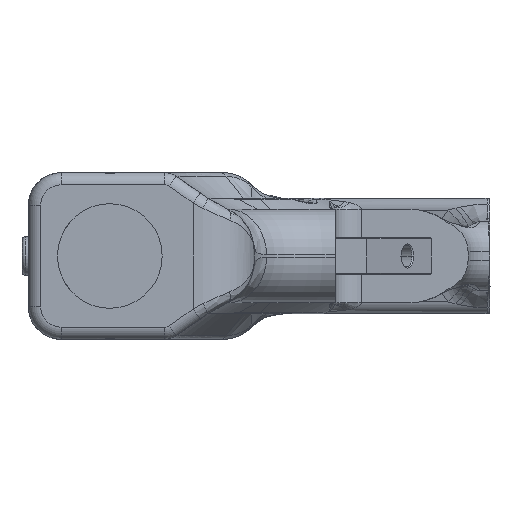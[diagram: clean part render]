
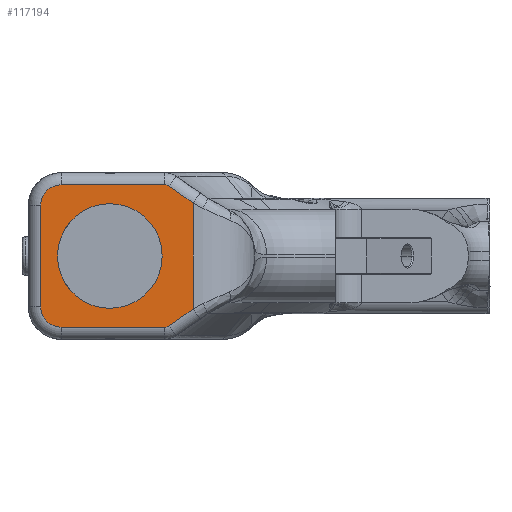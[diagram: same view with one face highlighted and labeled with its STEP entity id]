
A CAD part, left-side view. The second image highlights one B-rep face of the part: STEP entity #117194.
In plain terms, the highlighted planar face has unit normal (-1, 0, 0).
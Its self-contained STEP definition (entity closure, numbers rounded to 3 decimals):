
#360 = DIRECTION ( 'NONE',  ( 0., 0., 1. ) ) ;
#1329 = LINE ( 'NONE', #1911, #47660 ) ;
#1911 = CARTESIAN_POINT ( 'NONE',  ( -114.956, 0., -17.5 ) ) ;
#2619 = ORIENTED_EDGE ( 'NONE', *, *, #18241, .T. ) ;
#3771 = VECTOR ( 'NONE', #27679, 1000. ) ;
#4796 = ORIENTED_EDGE ( 'NONE', *, *, #19555, .T. ) ;
#6329 = CARTESIAN_POINT ( 'NONE',  ( -114.956, 105.1, -12.5 ) ) ;
#7355 = ORIENTED_EDGE ( 'NONE', *, *, #96632, .F. ) ;
#7951 = AXIS2_PLACEMENT_3D ( 'NONE', #50968, #42024, #105736 ) ;
#9005 = CARTESIAN_POINT ( 'NONE',  ( -114.956, 0., 20.5 ) ) ;
#9691 = ORIENTED_EDGE ( 'NONE', *, *, #30920, .T. ) ;
#10786 = CARTESIAN_POINT ( 'NONE',  ( -114.956, 69.321, -14.243 ) ) ;
#11739 = CARTESIAN_POINT ( 'NONE',  ( -114.956, 100.1, 12.5 ) ) ;
#11894 = CIRCLE ( 'NONE', #78513, 5. ) ;
#12187 = CIRCLE ( 'NONE', #109183, 12.875 ) ;
#14694 = LINE ( 'NONE', #106394, #98875 ) ;
#15686 = VECTOR ( 'NONE', #18559, 1000. ) ;
#16427 = ORIENTED_EDGE ( 'NONE', *, *, #97633, .F. ) ;
#16458 = DIRECTION ( 'NONE',  ( 0., 0., -1. ) ) ;
#16618 = AXIS2_PLACEMENT_3D ( 'NONE', #9005, #44818, #107895 ) ;
#17381 = ORIENTED_EDGE ( 'NONE', *, *, #26179, .T. ) ;
#17707 = DIRECTION ( 'NONE',  ( -1., 0., 0. ) ) ;
#18241 = EDGE_CURVE ( 'NONE', #76110, #98647, #51787, .T. ) ;
#18559 = DIRECTION ( 'NONE',  ( 0., -0.819, 0.574 ) ) ;
#19555 = EDGE_CURVE ( 'NONE', #110457, #112141, #101344, .T. ) ;
#22358 = DIRECTION ( 'NONE',  ( 0., 0., 1. ) ) ;
#22419 = DIRECTION ( 'NONE',  ( -1., 0., 0. ) ) ;
#26179 = EDGE_CURVE ( 'NONE', #66870, #110457, #110592, .T. ) ;
#26404 = CARTESIAN_POINT ( 'NONE',  ( -114.956, 74.602, -17.5 ) ) ;
#27619 = CARTESIAN_POINT ( 'NONE',  ( -114.956, 67.6, 13.038 ) ) ;
#27635 = ORIENTED_EDGE ( 'NONE', *, *, #94791, .F. ) ;
#27679 = DIRECTION ( 'NONE',  ( 0., 1., 0. ) ) ;
#28690 = CIRCLE ( 'NONE', #49685, 12.875 ) ;
#30236 = LINE ( 'NONE', #49335, #41963 ) ;
#30920 = EDGE_CURVE ( 'NONE', #75499, #31931, #11894, .T. ) ;
#31931 = VERTEX_POINT ( 'NONE', #103883 ) ;
#33222 = ORIENTED_EDGE ( 'NONE', *, *, #55880, .T. ) ;
#36606 = LINE ( 'NONE', #72950, #3771 ) ;
#37031 = CARTESIAN_POINT ( 'NONE',  ( -114.956, 88.1, 12.875 ) ) ;
#38508 = CARTESIAN_POINT ( 'NONE',  ( -114.956, 88.1, 0. ) ) ;
#38615 = DIRECTION ( 'NONE',  ( 0., 0.819, 0.574 ) ) ;
#40688 = LINE ( 'NONE', #41837, #67147 ) ;
#41305 = DIRECTION ( 'NONE',  ( -1., 0., 0. ) ) ;
#41555 = EDGE_CURVE ( 'NONE', #98647, #66870, #1329, .T. ) ;
#41837 = CARTESIAN_POINT ( 'NONE',  ( -114.956, 105.1, 20.5 ) ) ;
#41963 = VECTOR ( 'NONE', #38615, 1000. ) ;
#42024 = DIRECTION ( 'NONE',  ( -1., 0., 0. ) ) ;
#42637 = CARTESIAN_POINT ( 'NONE',  ( -114.956, 88.1, -12.875 ) ) ;
#44818 = DIRECTION ( 'NONE',  ( 1., 0., 0. ) ) ;
#46536 = EDGE_CURVE ( 'NONE', #31931, #76110, #40688, .T. ) ;
#47660 = VECTOR ( 'NONE', #100260, 1000. ) ;
#49335 = CARTESIAN_POINT ( 'NONE',  ( -114.956, 73.455, 17.138 ) ) ;
#49685 = AXIS2_PLACEMENT_3D ( 'NONE', #38508, #17707, #360 ) ;
#50829 = ORIENTED_EDGE ( 'NONE', *, *, #86669, .T. ) ;
#50968 = CARTESIAN_POINT ( 'NONE',  ( -114.956, 100.1, -12.5 ) ) ;
#51787 = CIRCLE ( 'NONE', #7951, 5. ) ;
#52511 = VERTEX_POINT ( 'NONE', #42637 ) ;
#54328 = FACE_OUTER_BOUND ( 'NONE', #108812, .T. ) ;
#55880 = EDGE_CURVE ( 'NONE', #89322, #75499, #36606, .T. ) ;
#56351 = VERTEX_POINT ( 'NONE', #95979 ) ;
#58770 = DIRECTION ( 'NONE',  ( 0., 0., -1. ) ) ;
#58804 = EDGE_LOOP ( 'NONE', ( #27635, #7355 ) ) ;
#65237 = ORIENTED_EDGE ( 'NONE', *, *, #41555, .T. ) ;
#66530 = DIRECTION ( 'NONE',  ( 0., 0., -1. ) ) ;
#66870 = VERTEX_POINT ( 'NONE', #26404 ) ;
#67147 = VECTOR ( 'NONE', #113297, 1000. ) ;
#67703 = CARTESIAN_POINT ( 'NONE',  ( -114.956, 74.602, 17.5 ) ) ;
#69094 = VERTEX_POINT ( 'NONE', #27619 ) ;
#71618 = FACE_BOUND ( 'NONE', #58804, .T. ) ;
#72950 = CARTESIAN_POINT ( 'NONE',  ( -114.956, 100.1, 17.5 ) ) ;
#73690 = CARTESIAN_POINT ( 'NONE',  ( -114.956, 100.1, 17.5 ) ) ;
#75499 = VERTEX_POINT ( 'NONE', #73690 ) ;
#76110 = VERTEX_POINT ( 'NONE', #6329 ) ;
#77280 = CIRCLE ( 'NONE', #84864, 2. ) ;
#78513 = AXIS2_PLACEMENT_3D ( 'NONE', #11739, #111760, #66530 ) ;
#78813 = DIRECTION ( 'NONE',  ( 0., 0., -1. ) ) ;
#84612 = VERTEX_POINT ( 'NONE', #37031 ) ;
#84864 = AXIS2_PLACEMENT_3D ( 'NONE', #86606, #41305, #78813 ) ;
#86606 = CARTESIAN_POINT ( 'NONE',  ( -114.956, 74.602, 15.5 ) ) ;
#86669 = EDGE_CURVE ( 'NONE', #69094, #56351, #30236, .T. ) ;
#89040 = CARTESIAN_POINT ( 'NONE',  ( -114.956, 73.455, -17.138 ) ) ;
#89322 = VERTEX_POINT ( 'NONE', #67703 ) ;
#89653 = ORIENTED_EDGE ( 'NONE', *, *, #102535, .T. ) ;
#90666 = PLANE ( 'NONE',  #16618 ) ;
#93308 = AXIS2_PLACEMENT_3D ( 'NONE', #93346, #22419, #58770 ) ;
#93346 = CARTESIAN_POINT ( 'NONE',  ( -114.956, 74.602, -15.5 ) ) ;
#94791 = EDGE_CURVE ( 'NONE', #84612, #52511, #12187, .T. ) ;
#95979 = CARTESIAN_POINT ( 'NONE',  ( -114.956, 73.455, 17.138 ) ) ;
#96632 = EDGE_CURVE ( 'NONE', #52511, #84612, #28690, .T. ) ;
#96781 = DIRECTION ( 'NONE',  ( -1., 0., 0. ) ) ;
#97633 = EDGE_CURVE ( 'NONE', #69094, #112141, #14694, .T. ) ;
#98647 = VERTEX_POINT ( 'NONE', #113611 ) ;
#98875 = VECTOR ( 'NONE', #16458, 1000. ) ;
#99856 = CARTESIAN_POINT ( 'NONE',  ( -114.956, 67.6, -13.038 ) ) ;
#100260 = DIRECTION ( 'NONE',  ( 0., -1., 0. ) ) ;
#101344 = LINE ( 'NONE', #10786, #15686 ) ;
#102535 = EDGE_CURVE ( 'NONE', #56351, #89322, #77280, .T. ) ;
#103883 = CARTESIAN_POINT ( 'NONE',  ( -114.956, 105.1, 12.5 ) ) ;
#105736 = DIRECTION ( 'NONE',  ( 0., 0., -1. ) ) ;
#106394 = CARTESIAN_POINT ( 'NONE',  ( -114.956, 67.6, 20.503 ) ) ;
#107895 = DIRECTION ( 'NONE',  ( 0., 0., -1. ) ) ;
#108812 = EDGE_LOOP ( 'NONE', ( #17381, #4796, #16427, #50829, #89653, #33222, #9691, #114010, #2619, #65237 ) ) ;
#109183 = AXIS2_PLACEMENT_3D ( 'NONE', #113447, #96781, #22358 ) ;
#110457 = VERTEX_POINT ( 'NONE', #89040 ) ;
#110592 = CIRCLE ( 'NONE', #93308, 2. ) ;
#111760 = DIRECTION ( 'NONE',  ( -1., 0., 0. ) ) ;
#112141 = VERTEX_POINT ( 'NONE', #99856 ) ;
#113297 = DIRECTION ( 'NONE',  ( 0., 0., -1. ) ) ;
#113447 = CARTESIAN_POINT ( 'NONE',  ( -114.956, 88.1, 0. ) ) ;
#113611 = CARTESIAN_POINT ( 'NONE',  ( -114.956, 100.1, -17.5 ) ) ;
#114010 = ORIENTED_EDGE ( 'NONE', *, *, #46536, .T. ) ;
#117194 = ADVANCED_FACE ( 'NONE', ( #71618, #54328 ), #90666, .F. ) ;
